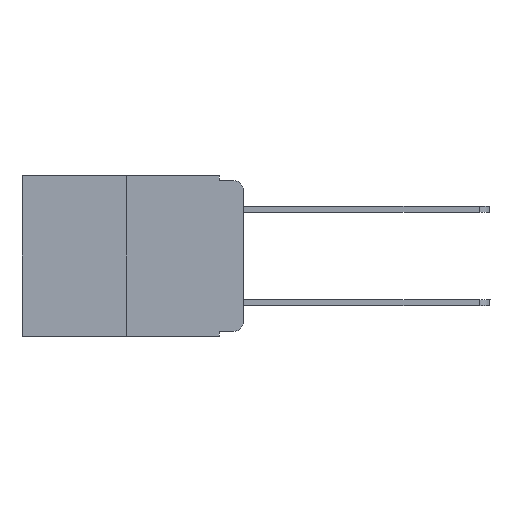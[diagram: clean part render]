
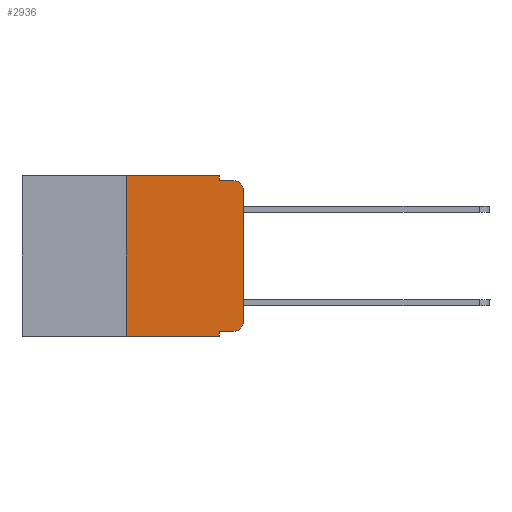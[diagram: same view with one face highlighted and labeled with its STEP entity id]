
A CAD part, left-side view. The second image highlights one B-rep face of the part: STEP entity #2936.
In plain terms, the highlighted planar face has unit normal (-1, 0, 0).
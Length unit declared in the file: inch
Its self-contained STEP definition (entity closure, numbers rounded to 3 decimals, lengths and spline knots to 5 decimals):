
#250 = EDGE_CURVE ( 'NONE', #2800, #13599, #3852, .T. ) ;
#319 = AXIS2_PLACEMENT_3D ( 'NONE', #9299, #15973, #14573 ) ;
#898 = PLANE ( 'NONE',  #13484 ) ;
#931 = DIRECTION ( 'NONE',  ( 0., -1., 0. ) ) ;
#1143 = VECTOR ( 'NONE', #931, 39.37008 ) ;
#1170 = FACE_OUTER_BOUND ( 'NONE', #3865, .T. ) ;
#1172 = CARTESIAN_POINT ( 'NONE',  ( 0., 0.051, -0.343 ) ) ;
#1174 = DIRECTION ( 'NONE',  ( 0., -1., 0. ) ) ;
#1286 = CARTESIAN_POINT ( 'NONE',  ( 0., 0.051, -0.01 ) ) ;
#2021 = DIRECTION ( 'NONE',  ( 0., 0., -1. ) ) ;
#2051 = CARTESIAN_POINT ( 'NONE',  ( 0., 0.02, -0.333 ) ) ;
#2083 = ORIENTED_EDGE ( 'NONE', *, *, #250, .F. ) ;
#2374 = DIRECTION ( 'NONE',  ( 0., -1., 0. ) ) ;
#2457 = LINE ( 'NONE', #17049, #16346 ) ;
#2504 = AXIS2_PLACEMENT_3D ( 'NONE', #13715, #7186, #2021 ) ;
#2759 = DIRECTION ( 'NONE',  ( 0., -1., 0. ) ) ;
#2800 = VERTEX_POINT ( 'NONE', #2811 ) ;
#2811 = CARTESIAN_POINT ( 'NONE',  ( 0., 0.25, -0.343 ) ) ;
#2867 = EDGE_CURVE ( 'NONE', #4944, #10801, #5794, .T. ) ;
#2936 = ADVANCED_FACE ( 'NONE', ( #1170 ), #898, .F. ) ;
#3511 = EDGE_CURVE ( 'NONE', #6432, #7678, #8794, .T. ) ;
#3580 = ORIENTED_EDGE ( 'NONE', *, *, #4482, .T. ) ;
#3599 = ORIENTED_EDGE ( 'NONE', *, *, #3511, .F. ) ;
#3630 = CIRCLE ( 'NONE', #319, 0.02 ) ;
#3677 = CARTESIAN_POINT ( 'NONE',  ( 0., 0.473, -0.343 ) ) ;
#3780 = CARTESIAN_POINT ( 'NONE',  ( 0., 0., -0.313 ) ) ;
#3852 = LINE ( 'NONE', #13125, #5160 ) ;
#3865 = EDGE_LOOP ( 'NONE', ( #13515, #3580, #4218, #3599, #12292, #2083, #14790, #4044, #13483, #13944 ) ) ;
#4018 = DIRECTION ( 'NONE',  ( 0., 0., 1. ) ) ;
#4044 = ORIENTED_EDGE ( 'NONE', *, *, #14760, .F. ) ;
#4102 = CARTESIAN_POINT ( 'NONE',  ( 0., 0.051, -0.01 ) ) ;
#4218 = ORIENTED_EDGE ( 'NONE', *, *, #10833, .F. ) ;
#4309 = EDGE_CURVE ( 'NONE', #2800, #13507, #15489, .T. ) ;
#4482 = EDGE_CURVE ( 'NONE', #12575, #8884, #3630, .T. ) ;
#4828 = CARTESIAN_POINT ( 'NONE',  ( 0., 0., -0.03 ) ) ;
#4944 = VERTEX_POINT ( 'NONE', #2051 ) ;
#5160 = VECTOR ( 'NONE', #4018, 39.37008 ) ;
#5794 = CIRCLE ( 'NONE', #2504, 0.02 ) ;
#6432 = VERTEX_POINT ( 'NONE', #16867 ) ;
#7165 = CARTESIAN_POINT ( 'NONE',  ( 0., 0., 0. ) ) ;
#7186 = DIRECTION ( 'NONE',  ( -1., 0., 0. ) ) ;
#7678 = VERTEX_POINT ( 'NONE', #4102 ) ;
#7714 = CARTESIAN_POINT ( 'NONE',  ( 0., 0.473, 0. ) ) ;
#7814 = VECTOR ( 'NONE', #7972, 39.37008 ) ;
#7916 = CARTESIAN_POINT ( 'NONE',  ( 0., 0.051, -0.333 ) ) ;
#7972 = DIRECTION ( 'NONE',  ( 0., 0., -1. ) ) ;
#8246 = LINE ( 'NONE', #9284, #10075 ) ;
#8513 = EDGE_CURVE ( 'NONE', #10801, #12575, #11479, .T. ) ;
#8537 = DIRECTION ( 'NONE',  ( 0., 0., 1. ) ) ;
#8794 = LINE ( 'NONE', #15357, #9370 ) ;
#8884 = VERTEX_POINT ( 'NONE', #14030 ) ;
#9284 = CARTESIAN_POINT ( 'NONE',  ( 0., 0.051, -0.333 ) ) ;
#9293 = EDGE_CURVE ( 'NONE', #10883, #4944, #8246, .T. ) ;
#9299 = CARTESIAN_POINT ( 'NONE',  ( 0., 0.02, -0.03 ) ) ;
#9370 = VECTOR ( 'NONE', #14049, 39.37008 ) ;
#9490 = CARTESIAN_POINT ( 'NONE',  ( 0., 0.25, 0. ) ) ;
#10075 = VECTOR ( 'NONE', #2759, 39.37008 ) ;
#10455 = DIRECTION ( 'NONE',  ( 1., 0., 0. ) ) ;
#10801 = VERTEX_POINT ( 'NONE', #3780 ) ;
#10833 = EDGE_CURVE ( 'NONE', #7678, #8884, #13066, .T. ) ;
#10883 = VERTEX_POINT ( 'NONE', #7916 ) ;
#11047 = VECTOR ( 'NONE', #2374, 39.37008 ) ;
#11479 = LINE ( 'NONE', #7165, #14786 ) ;
#12292 = ORIENTED_EDGE ( 'NONE', *, *, #14739, .F. ) ;
#12575 = VERTEX_POINT ( 'NONE', #4828 ) ;
#12941 = DIRECTION ( 'NONE',  ( 0., 0., -1. ) ) ;
#13066 = LINE ( 'NONE', #1286, #1143 ) ;
#13125 = CARTESIAN_POINT ( 'NONE',  ( 0., 0.25, 0. ) ) ;
#13483 = ORIENTED_EDGE ( 'NONE', *, *, #9293, .T. ) ;
#13484 = AXIS2_PLACEMENT_3D ( 'NONE', #7714, #10455, #12941 ) ;
#13507 = VERTEX_POINT ( 'NONE', #1172 ) ;
#13515 = ORIENTED_EDGE ( 'NONE', *, *, #8513, .T. ) ;
#13599 = VERTEX_POINT ( 'NONE', #9490 ) ;
#13715 = CARTESIAN_POINT ( 'NONE',  ( 0., 0.02, -0.313 ) ) ;
#13944 = ORIENTED_EDGE ( 'NONE', *, *, #2867, .T. ) ;
#14030 = CARTESIAN_POINT ( 'NONE',  ( 0., 0.02, -0.01 ) ) ;
#14049 = DIRECTION ( 'NONE',  ( 0., 0., -1. ) ) ;
#14252 = CARTESIAN_POINT ( 'NONE',  ( 0., 0.051, 0. ) ) ;
#14573 = DIRECTION ( 'NONE',  ( 0., 0., -1. ) ) ;
#14739 = EDGE_CURVE ( 'NONE', #13599, #6432, #2457, .T. ) ;
#14760 = EDGE_CURVE ( 'NONE', #10883, #13507, #15748, .T. ) ;
#14786 = VECTOR ( 'NONE', #8537, 39.37008 ) ;
#14790 = ORIENTED_EDGE ( 'NONE', *, *, #4309, .T. ) ;
#15357 = CARTESIAN_POINT ( 'NONE',  ( 0., 0.051, 0. ) ) ;
#15489 = LINE ( 'NONE', #3677, #11047 ) ;
#15748 = LINE ( 'NONE', #14252, #7814 ) ;
#15973 = DIRECTION ( 'NONE',  ( -1., 0., 0. ) ) ;
#16346 = VECTOR ( 'NONE', #1174, 39.37008 ) ;
#16867 = CARTESIAN_POINT ( 'NONE',  ( 0., 0.051, 0. ) ) ;
#17049 = CARTESIAN_POINT ( 'NONE',  ( 0., 0.473, 0. ) ) ;
